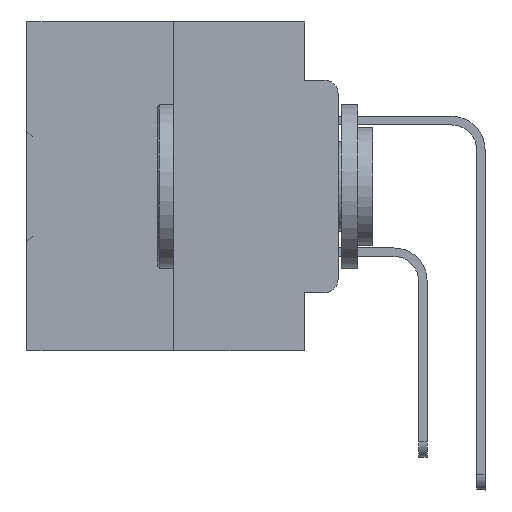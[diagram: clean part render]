
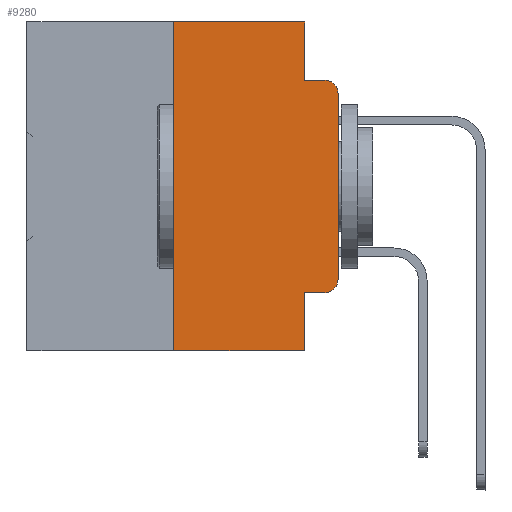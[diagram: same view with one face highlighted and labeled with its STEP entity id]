
A CAD part, left-side view. The second image highlights one B-rep face of the part: STEP entity #9280.
In plain terms, the highlighted planar face has unit normal (-1, 0, 0).
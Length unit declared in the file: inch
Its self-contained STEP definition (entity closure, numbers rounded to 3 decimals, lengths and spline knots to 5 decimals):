
#202 = DIRECTION ( 'NONE',  ( 0., 0., -1. ) ) ;
#1008 = LINE ( 'NONE', #1196, #22558 ) ;
#1057 = CARTESIAN_POINT ( 'NONE',  ( 0., 0.473, 0. ) ) ;
#1196 = CARTESIAN_POINT ( 'NONE',  ( 0., 0.473, -0.5 ) ) ;
#1246 = CARTESIAN_POINT ( 'NONE',  ( 0., 0.051, -0.0885 ) ) ;
#2184 = CARTESIAN_POINT ( 'NONE',  ( 0., 0.25, 0. ) ) ;
#2518 = DIRECTION ( 'NONE',  ( -1., 0., 0. ) ) ;
#2862 = EDGE_CURVE ( 'NONE', #15620, #9601, #1008, .T. ) ;
#3117 = ORIENTED_EDGE ( 'NONE', *, *, #3722, .T. ) ;
#3360 = VERTEX_POINT ( 'NONE', #1246 ) ;
#3579 = ORIENTED_EDGE ( 'NONE', *, *, #12634, .F. ) ;
#3722 = EDGE_CURVE ( 'NONE', #12328, #17885, #9021, .T. ) ;
#4555 = CARTESIAN_POINT ( 'NONE',  ( 0., 0.25, 0. ) ) ;
#4830 = CARTESIAN_POINT ( 'NONE',  ( 0., 0.02, -0.0885 ) ) ;
#5282 = EDGE_CURVE ( 'NONE', #32154, #24292, #6515, .T. ) ;
#5922 = CARTESIAN_POINT ( 'NONE',  ( 0., 0.02, -0.3915 ) ) ;
#6515 = CIRCLE ( 'NONE', #10759, 0.02 ) ;
#6743 = DIRECTION ( 'NONE',  ( 0., -1., 0. ) ) ;
#7398 = LINE ( 'NONE', #4555, #10306 ) ;
#7473 = CARTESIAN_POINT ( 'NONE',  ( 0., 0.051, 0. ) ) ;
#7717 = LINE ( 'NONE', #1057, #10434 ) ;
#8266 = VERTEX_POINT ( 'NONE', #2184 ) ;
#8549 = VERTEX_POINT ( 'NONE', #7473 ) ;
#8705 = DIRECTION ( 'NONE',  ( 0., 0., -1. ) ) ;
#9021 = LINE ( 'NONE', #15086, #29937 ) ;
#9037 = LINE ( 'NONE', #17768, #15357 ) ;
#9280 = ADVANCED_FACE ( 'NONE', ( #25269 ), #36873, .F. ) ;
#9601 = VERTEX_POINT ( 'NONE', #19508 ) ;
#10192 = ORIENTED_EDGE ( 'NONE', *, *, #18291, .F. ) ;
#10306 = VECTOR ( 'NONE', #27899, 39.37008 ) ;
#10354 = ORIENTED_EDGE ( 'NONE', *, *, #19421, .F. ) ;
#10434 = VECTOR ( 'NONE', #12666, 39.37008 ) ;
#10759 = AXIS2_PLACEMENT_3D ( 'NONE', #29384, #17221, #12271 ) ;
#10820 = DIRECTION ( 'NONE',  ( 0., 0., -1. ) ) ;
#10907 = EDGE_CURVE ( 'NONE', #8266, #8549, #7717, .T. ) ;
#11494 = EDGE_CURVE ( 'NONE', #22418, #32154, #22275, .T. ) ;
#12271 = DIRECTION ( 'NONE',  ( 0., 0., -1. ) ) ;
#12328 = VERTEX_POINT ( 'NONE', #24646 ) ;
#12634 = EDGE_CURVE ( 'NONE', #8549, #3360, #9037, .T. ) ;
#12666 = DIRECTION ( 'NONE',  ( 0., -1., 0. ) ) ;
#13293 = DIRECTION ( 'NONE',  ( 1., 0., 0. ) ) ;
#14322 = ORIENTED_EDGE ( 'NONE', *, *, #2862, .T. ) ;
#15086 = CARTESIAN_POINT ( 'NONE',  ( 0., 0.051, -0.4115 ) ) ;
#15357 = VECTOR ( 'NONE', #36564, 39.37008 ) ;
#15620 = VERTEX_POINT ( 'NONE', #24132 ) ;
#16146 = EDGE_LOOP ( 'NONE', ( #32183, #34283, #17982, #3579, #23997, #10354, #14322, #10192, #3117, #24865 ) ) ;
#16200 = CARTESIAN_POINT ( 'NONE',  ( 0., 0., -0.1085 ) ) ;
#17221 = DIRECTION ( 'NONE',  ( -1., 0., 0. ) ) ;
#17768 = CARTESIAN_POINT ( 'NONE',  ( 0., 0.051, 0. ) ) ;
#17885 = VERTEX_POINT ( 'NONE', #19841 ) ;
#17982 = ORIENTED_EDGE ( 'NONE', *, *, #29777, .F. ) ;
#18291 = EDGE_CURVE ( 'NONE', #12328, #9601, #25977, .T. ) ;
#19254 = DIRECTION ( 'NONE',  ( 0., 0., 1. ) ) ;
#19421 = EDGE_CURVE ( 'NONE', #15620, #8266, #7398, .T. ) ;
#19508 = CARTESIAN_POINT ( 'NONE',  ( 0., 0.051, -0.5 ) ) ;
#19540 = VECTOR ( 'NONE', #19254, 39.37008 ) ;
#19841 = CARTESIAN_POINT ( 'NONE',  ( 0., 0.02, -0.4115 ) ) ;
#22275 = LINE ( 'NONE', #28365, #19540 ) ;
#22418 = VERTEX_POINT ( 'NONE', #29593 ) ;
#22558 = VECTOR ( 'NONE', #6743, 39.37008 ) ;
#22776 = CIRCLE ( 'NONE', #24625, 0.02 ) ;
#23997 = ORIENTED_EDGE ( 'NONE', *, *, #10907, .F. ) ;
#24132 = CARTESIAN_POINT ( 'NONE',  ( 0., 0.25, -0.5 ) ) ;
#24292 = VERTEX_POINT ( 'NONE', #4830 ) ;
#24625 = AXIS2_PLACEMENT_3D ( 'NONE', #5922, #2518, #202 ) ;
#24646 = CARTESIAN_POINT ( 'NONE',  ( 0., 0.051, -0.4115 ) ) ;
#24865 = ORIENTED_EDGE ( 'NONE', *, *, #28522, .T. ) ;
#24894 = CARTESIAN_POINT ( 'NONE',  ( 0., 0.473, 0. ) ) ;
#25269 = FACE_OUTER_BOUND ( 'NONE', #16146, .T. ) ;
#25479 = AXIS2_PLACEMENT_3D ( 'NONE', #24894, #13293, #10820 ) ;
#25977 = LINE ( 'NONE', #37587, #29656 ) ;
#26442 = LINE ( 'NONE', #28742, #32042 ) ;
#27899 = DIRECTION ( 'NONE',  ( 0., 0., 1. ) ) ;
#28365 = CARTESIAN_POINT ( 'NONE',  ( 0., 0., 0. ) ) ;
#28522 = EDGE_CURVE ( 'NONE', #17885, #22418, #22776, .T. ) ;
#28742 = CARTESIAN_POINT ( 'NONE',  ( 0., 0.051, -0.0885 ) ) ;
#29112 = DIRECTION ( 'NONE',  ( 0., -1., 0. ) ) ;
#29384 = CARTESIAN_POINT ( 'NONE',  ( 0., 0.02, -0.1085 ) ) ;
#29593 = CARTESIAN_POINT ( 'NONE',  ( 0., 0., -0.3915 ) ) ;
#29656 = VECTOR ( 'NONE', #8705, 39.37008 ) ;
#29777 = EDGE_CURVE ( 'NONE', #3360, #24292, #26442, .T. ) ;
#29937 = VECTOR ( 'NONE', #32210, 39.37008 ) ;
#32042 = VECTOR ( 'NONE', #29112, 39.37008 ) ;
#32154 = VERTEX_POINT ( 'NONE', #16200 ) ;
#32183 = ORIENTED_EDGE ( 'NONE', *, *, #11494, .T. ) ;
#32210 = DIRECTION ( 'NONE',  ( 0., -1., 0. ) ) ;
#34283 = ORIENTED_EDGE ( 'NONE', *, *, #5282, .T. ) ;
#36564 = DIRECTION ( 'NONE',  ( 0., 0., -1. ) ) ;
#36873 = PLANE ( 'NONE',  #25479 ) ;
#37587 = CARTESIAN_POINT ( 'NONE',  ( 0., 0.051, 0. ) ) ;
